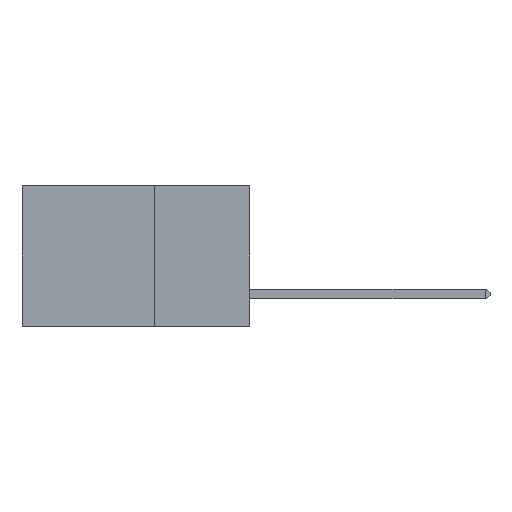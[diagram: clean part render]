
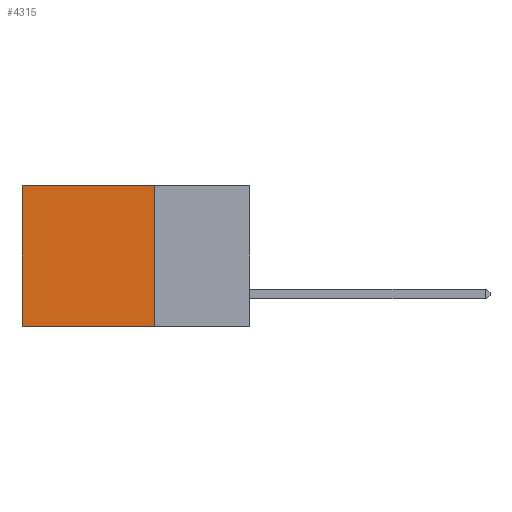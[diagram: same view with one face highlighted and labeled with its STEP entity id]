
A CAD part, left-side view. The second image highlights one B-rep face of the part: STEP entity #4315.
In plain terms, the highlighted planar face has unit normal (-1, 0, 0).
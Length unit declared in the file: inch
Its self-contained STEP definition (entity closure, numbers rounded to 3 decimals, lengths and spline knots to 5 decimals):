
#551 = CARTESIAN_POINT ( 'NONE',  ( 0.2875, 0.25, -0.37 ) ) ;
#1303 = LINE ( 'NONE', #15566, #6279 ) ;
#1388 = VERTEX_POINT ( 'NONE', #10862 ) ;
#4315 = ADVANCED_FACE ( 'NONE', ( #12189 ), #22017, .F. ) ;
#5306 = DIRECTION ( 'NONE',  ( 0., 0., -1. ) ) ;
#5511 = DIRECTION ( 'NONE',  ( 0., 1., 0. ) ) ;
#5590 = VECTOR ( 'NONE', #5306, 39.37008 ) ;
#5725 = DIRECTION ( 'NONE',  ( 0., 0., -1. ) ) ;
#6279 = VECTOR ( 'NONE', #5511, 39.37008 ) ;
#6942 = AXIS2_PLACEMENT_3D ( 'NONE', #23981, #25895, #14200 ) ;
#8442 = ORIENTED_EDGE ( 'NONE', *, *, #20933, .F. ) ;
#8523 = VECTOR ( 'NONE', #12985, 39.37008 ) ;
#8976 = ORIENTED_EDGE ( 'NONE', *, *, #21417, .F. ) ;
#10862 = CARTESIAN_POINT ( 'NONE',  ( 0.2875, 0.25, -0.37 ) ) ;
#12189 = FACE_OUTER_BOUND ( 'NONE', #17418, .T. ) ;
#12474 = ORIENTED_EDGE ( 'NONE', *, *, #20479, .T. ) ;
#12622 = VECTOR ( 'NONE', #5725, 39.37008 ) ;
#12985 = DIRECTION ( 'NONE',  ( 0., 1., 0. ) ) ;
#14200 = DIRECTION ( 'NONE',  ( 0., 0., -1. ) ) ;
#14422 = LINE ( 'NONE', #551, #8523 ) ;
#14802 = CARTESIAN_POINT ( 'NONE',  ( 0.2875, 0.6, -0.37 ) ) ;
#15058 = LINE ( 'NONE', #17354, #5590 ) ;
#15566 = CARTESIAN_POINT ( 'NONE',  ( 0.2875, 0.25, 0. ) ) ;
#15853 = VERTEX_POINT ( 'NONE', #22586 ) ;
#16483 = VERTEX_POINT ( 'NONE', #23863 ) ;
#17200 = VERTEX_POINT ( 'NONE', #14802 ) ;
#17354 = CARTESIAN_POINT ( 'NONE',  ( 0.2875, 0.25, 0. ) ) ;
#17418 = EDGE_LOOP ( 'NONE', ( #20360, #8976, #8442, #12474 ) ) ;
#17823 = LINE ( 'NONE', #19704, #12622 ) ;
#19704 = CARTESIAN_POINT ( 'NONE',  ( 0.2875, 0.6, 0. ) ) ;
#20360 = ORIENTED_EDGE ( 'NONE', *, *, #24851, .T. ) ;
#20479 = EDGE_CURVE ( 'NONE', #15853, #16483, #1303, .T. ) ;
#20933 = EDGE_CURVE ( 'NONE', #15853, #1388, #15058, .T. ) ;
#21417 = EDGE_CURVE ( 'NONE', #1388, #17200, #14422, .T. ) ;
#22017 = PLANE ( 'NONE',  #6942 ) ;
#22586 = CARTESIAN_POINT ( 'NONE',  ( 0.2875, 0.25, 0. ) ) ;
#23863 = CARTESIAN_POINT ( 'NONE',  ( 0.2875, 0.6, 0. ) ) ;
#23981 = CARTESIAN_POINT ( 'NONE',  ( 0.2875, 0.25, 0. ) ) ;
#24851 = EDGE_CURVE ( 'NONE', #16483, #17200, #17823, .T. ) ;
#25895 = DIRECTION ( 'NONE',  ( 1., 0., 0. ) ) ;
